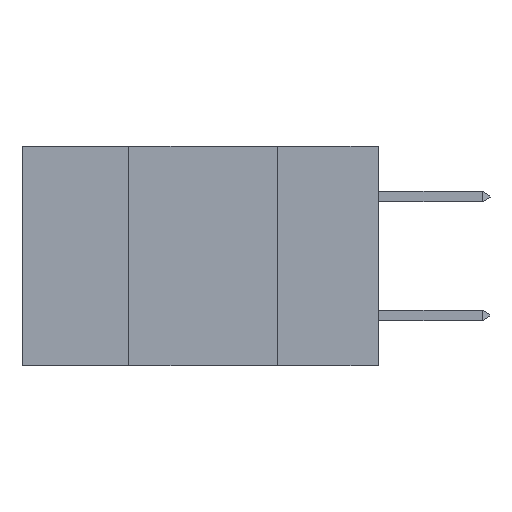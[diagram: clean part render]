
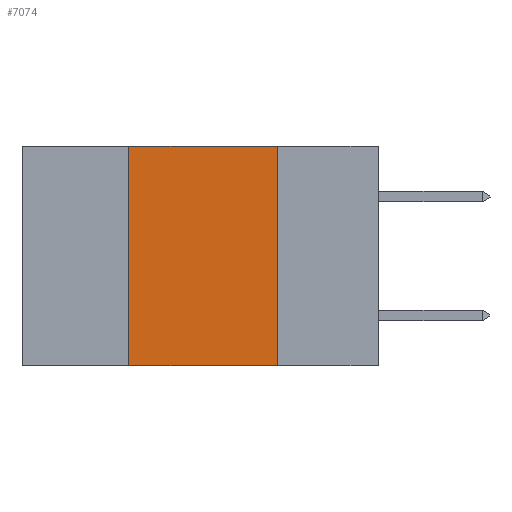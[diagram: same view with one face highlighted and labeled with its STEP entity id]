
A CAD part, left-side view. The second image highlights one B-rep face of the part: STEP entity #7074.
In plain terms, the highlighted planar face has unit normal (-1, 0, 0).
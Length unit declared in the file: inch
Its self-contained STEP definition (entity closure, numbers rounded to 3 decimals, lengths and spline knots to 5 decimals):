
#386 = VERTEX_POINT ( 'NONE', #28448 ) ;
#817 = CARTESIAN_POINT ( 'NONE',  ( 0., 0.42, 0. ) ) ;
#1297 = DIRECTION ( 'NONE',  ( 0., 0., -1. ) ) ;
#1995 = LINE ( 'NONE', #7444, #3966 ) ;
#2062 = ORIENTED_EDGE ( 'NONE', *, *, #19056, .F. ) ;
#3966 = VECTOR ( 'NONE', #9627, 39.37008 ) ;
#4808 = LINE ( 'NONE', #17799, #30080 ) ;
#5019 = ORIENTED_EDGE ( 'NONE', *, *, #11284, .F. ) ;
#7074 = ADVANCED_FACE ( 'NONE', ( #16668 ), #13774, .F. ) ;
#7444 = CARTESIAN_POINT ( 'NONE',  ( 0., 0.6, 0. ) ) ;
#9530 = ORIENTED_EDGE ( 'NONE', *, *, #24956, .F. ) ;
#9627 = DIRECTION ( 'NONE',  ( 0., -1., 0. ) ) ;
#11284 = EDGE_CURVE ( 'NONE', #16525, #24295, #31732, .T. ) ;
#11564 = VECTOR ( 'NONE', #26101, 39.37008 ) ;
#12498 = LINE ( 'NONE', #14581, #15272 ) ;
#13758 = VERTEX_POINT ( 'NONE', #16746 ) ;
#13774 = PLANE ( 'NONE',  #24456 ) ;
#14581 = CARTESIAN_POINT ( 'NONE',  ( 0., 0.6, -0.37 ) ) ;
#15272 = VECTOR ( 'NONE', #27377, 39.37008 ) ;
#16437 = DIRECTION ( 'NONE',  ( 1., 0., 0. ) ) ;
#16525 = VERTEX_POINT ( 'NONE', #18959 ) ;
#16668 = FACE_OUTER_BOUND ( 'NONE', #31383, .T. ) ;
#16746 = CARTESIAN_POINT ( 'NONE',  ( 0., 0.17, 0. ) ) ;
#17799 = CARTESIAN_POINT ( 'NONE',  ( 0., 0.17, 0. ) ) ;
#18959 = CARTESIAN_POINT ( 'NONE',  ( 0., 0.42, -0.37 ) ) ;
#19056 = EDGE_CURVE ( 'NONE', #13758, #386, #4808, .T. ) ;
#20537 = CARTESIAN_POINT ( 'NONE',  ( 0., 0.42, 0. ) ) ;
#21166 = EDGE_CURVE ( 'NONE', #16525, #386, #12498, .T. ) ;
#24295 = VERTEX_POINT ( 'NONE', #20537 ) ;
#24456 = AXIS2_PLACEMENT_3D ( 'NONE', #26461, #16437, #1297 ) ;
#24956 = EDGE_CURVE ( 'NONE', #24295, #13758, #1995, .T. ) ;
#26101 = DIRECTION ( 'NONE',  ( 0., 0., 1. ) ) ;
#26461 = CARTESIAN_POINT ( 'NONE',  ( 0., 0.6, 0. ) ) ;
#27377 = DIRECTION ( 'NONE',  ( 0., -1., 0. ) ) ;
#27486 = DIRECTION ( 'NONE',  ( 0., 0., -1. ) ) ;
#28448 = CARTESIAN_POINT ( 'NONE',  ( 0., 0.17, -0.37 ) ) ;
#30080 = VECTOR ( 'NONE', #27486, 39.37008 ) ;
#30577 = ORIENTED_EDGE ( 'NONE', *, *, #21166, .T. ) ;
#31383 = EDGE_LOOP ( 'NONE', ( #2062, #9530, #5019, #30577 ) ) ;
#31732 = LINE ( 'NONE', #817, #11564 ) ;
